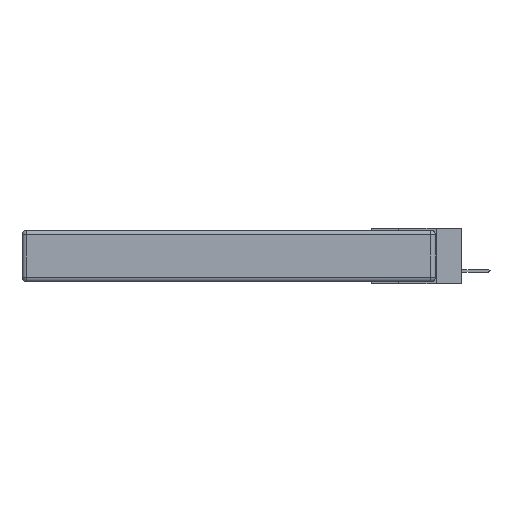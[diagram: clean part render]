
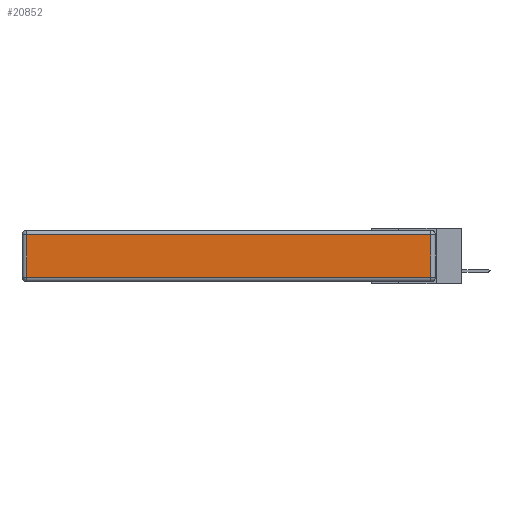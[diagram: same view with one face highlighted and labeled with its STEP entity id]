
A CAD part, left-side view. The second image highlights one B-rep face of the part: STEP entity #20852.
In plain terms, the highlighted planar face has unit normal (-1, 0, 0).
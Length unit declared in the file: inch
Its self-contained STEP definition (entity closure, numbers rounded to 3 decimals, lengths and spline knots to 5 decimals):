
#12 = EDGE_CURVE ( 'NONE', #1959, #3962, #2969, .T. ) ;
#91 = DIRECTION ( 'NONE',  ( 0., 0., 1. ) ) ;
#138 = FACE_OUTER_BOUND ( 'NONE', #9802, .T. ) ;
#922 = CARTESIAN_POINT ( 'NONE',  ( 0., 2.72, -0.313 ) ) ;
#1276 = ORIENTED_EDGE ( 'NONE', *, *, #20130, .T. ) ;
#1462 = EDGE_CURVE ( 'NONE', #13492, #20307, #11883, .T. ) ;
#1773 = LINE ( 'NONE', #2404, #14709 ) ;
#1959 = VERTEX_POINT ( 'NONE', #2802 ) ;
#2404 = CARTESIAN_POINT ( 'NONE',  ( 0., 2.75, -0.03 ) ) ;
#2802 = CARTESIAN_POINT ( 'NONE',  ( 0., 0.03, -0.313 ) ) ;
#2969 = LINE ( 'NONE', #15734, #16761 ) ;
#3962 = VERTEX_POINT ( 'NONE', #20312 ) ;
#5036 = PLANE ( 'NONE',  #9655 ) ;
#9655 = AXIS2_PLACEMENT_3D ( 'NONE', #15005, #18674, #91 ) ;
#9802 = EDGE_LOOP ( 'NONE', ( #18411, #19892, #1276, #13351 ) ) ;
#10207 = CARTESIAN_POINT ( 'NONE',  ( 0., 2.72, -0.03 ) ) ;
#10509 = CARTESIAN_POINT ( 'NONE',  ( 0., 2.72, -0.343 ) ) ;
#11883 = LINE ( 'NONE', #10509, #16399 ) ;
#12357 = DIRECTION ( 'NONE',  ( 0., 1., 0. ) ) ;
#12735 = DIRECTION ( 'NONE',  ( 0., -1., 0. ) ) ;
#13351 = ORIENTED_EDGE ( 'NONE', *, *, #1462, .T. ) ;
#13492 = VERTEX_POINT ( 'NONE', #10207 ) ;
#14709 = VECTOR ( 'NONE', #12357, 39.37008 ) ;
#15005 = CARTESIAN_POINT ( 'NONE',  ( 0., 0., -0.343 ) ) ;
#15031 = VECTOR ( 'NONE', #12735, 39.37008 ) ;
#15674 = DIRECTION ( 'NONE',  ( 0., 0., -1. ) ) ;
#15734 = CARTESIAN_POINT ( 'NONE',  ( 0., 0.03, -0.343 ) ) ;
#16399 = VECTOR ( 'NONE', #15674, 39.37008 ) ;
#16460 = CARTESIAN_POINT ( 'NONE',  ( 0., 0., -0.313 ) ) ;
#16761 = VECTOR ( 'NONE', #19419, 39.37008 ) ;
#16942 = LINE ( 'NONE', #16460, #15031 ) ;
#18411 = ORIENTED_EDGE ( 'NONE', *, *, #18630, .T. ) ;
#18630 = EDGE_CURVE ( 'NONE', #20307, #1959, #16942, .T. ) ;
#18674 = DIRECTION ( 'NONE',  ( -1., 0., 0. ) ) ;
#19419 = DIRECTION ( 'NONE',  ( 0., 0., 1. ) ) ;
#19892 = ORIENTED_EDGE ( 'NONE', *, *, #12, .T. ) ;
#20130 = EDGE_CURVE ( 'NONE', #3962, #13492, #1773, .T. ) ;
#20307 = VERTEX_POINT ( 'NONE', #922 ) ;
#20312 = CARTESIAN_POINT ( 'NONE',  ( 0., 0.03, -0.03 ) ) ;
#20852 = ADVANCED_FACE ( 'NONE', ( #138 ), #5036, .T. ) ;
